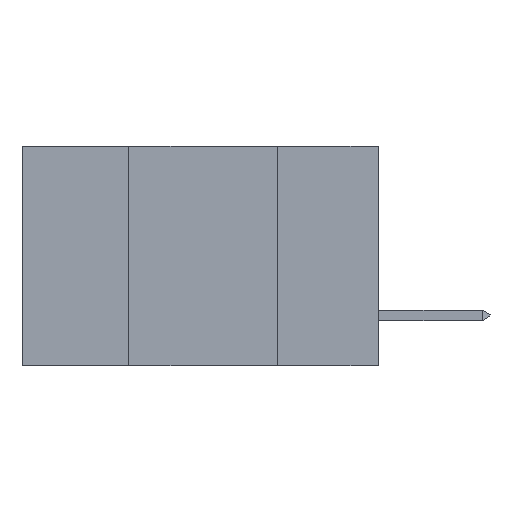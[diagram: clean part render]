
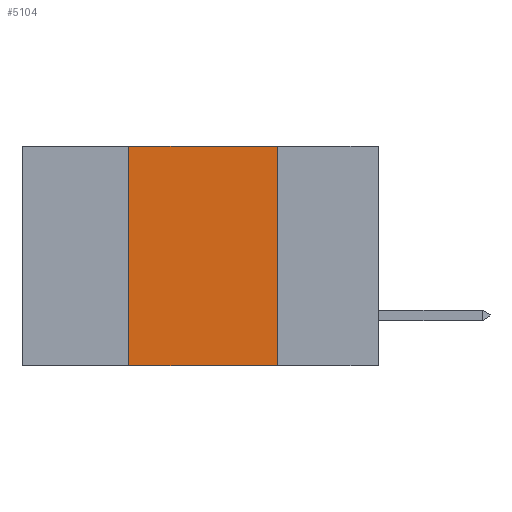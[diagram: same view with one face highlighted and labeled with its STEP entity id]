
A CAD part, left-side view. The second image highlights one B-rep face of the part: STEP entity #5104.
In plain terms, the highlighted planar face has unit normal (-1, 0, 0).
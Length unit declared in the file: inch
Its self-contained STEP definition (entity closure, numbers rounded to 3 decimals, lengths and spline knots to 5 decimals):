
#540 = EDGE_CURVE ( 'NONE', #7114, #6275, #2374, .T. ) ;
#1129 = AXIS2_PLACEMENT_3D ( 'NONE', #11163, #4843, #6060 ) ;
#2374 = LINE ( 'NONE', #8727, #5326 ) ;
#2601 = CARTESIAN_POINT ( 'NONE',  ( 0., 0.42, -0.37 ) ) ;
#2803 = CARTESIAN_POINT ( 'NONE',  ( 0., 0.17, -0.37 ) ) ;
#3100 = CARTESIAN_POINT ( 'NONE',  ( 0., 0.17, 0. ) ) ;
#3143 = DIRECTION ( 'NONE',  ( 0., -1., 0. ) ) ;
#3910 = DIRECTION ( 'NONE',  ( 0., 0., -1. ) ) ;
#4780 = VERTEX_POINT ( 'NONE', #3100 ) ;
#4843 = DIRECTION ( 'NONE',  ( 1., 0., 0. ) ) ;
#5104 = ADVANCED_FACE ( 'NONE', ( #5792 ), #13165, .F. ) ;
#5326 = VECTOR ( 'NONE', #11069, 39.37008 ) ;
#5466 = EDGE_CURVE ( 'NONE', #4780, #6275, #13154, .T. ) ;
#5792 = FACE_OUTER_BOUND ( 'NONE', #6506, .T. ) ;
#5858 = ORIENTED_EDGE ( 'NONE', *, *, #540, .T. ) ;
#6060 = DIRECTION ( 'NONE',  ( 0., 0., -1. ) ) ;
#6275 = VERTEX_POINT ( 'NONE', #13023 ) ;
#6387 = CARTESIAN_POINT ( 'NONE',  ( 0., 0.6, 0. ) ) ;
#6506 = EDGE_LOOP ( 'NONE', ( #10018, #6529, #9002, #5858 ) ) ;
#6529 = ORIENTED_EDGE ( 'NONE', *, *, #8451, .F. ) ;
#7114 = VERTEX_POINT ( 'NONE', #2601 ) ;
#7249 = CARTESIAN_POINT ( 'NONE',  ( 0., 0.42, -0.37 ) ) ;
#7506 = VERTEX_POINT ( 'NONE', #13211 ) ;
#8204 = LINE ( 'NONE', #6387, #9589 ) ;
#8451 = EDGE_CURVE ( 'NONE', #7506, #4780, #8204, .T. ) ;
#8727 = CARTESIAN_POINT ( 'NONE',  ( 0., 0.6, -0.37 ) ) ;
#9002 = ORIENTED_EDGE ( 'NONE', *, *, #12013, .F. ) ;
#9589 = VECTOR ( 'NONE', #3143, 39.37008 ) ;
#10018 = ORIENTED_EDGE ( 'NONE', *, *, #5466, .F. ) ;
#10231 = LINE ( 'NONE', #7249, #10305 ) ;
#10305 = VECTOR ( 'NONE', #12350, 39.37008 ) ;
#10861 = VECTOR ( 'NONE', #3910, 39.37008 ) ;
#11069 = DIRECTION ( 'NONE',  ( 0., -1., 0. ) ) ;
#11163 = CARTESIAN_POINT ( 'NONE',  ( 0., 0.6, 0. ) ) ;
#12013 = EDGE_CURVE ( 'NONE', #7114, #7506, #10231, .T. ) ;
#12350 = DIRECTION ( 'NONE',  ( 0., 0., 1. ) ) ;
#13023 = CARTESIAN_POINT ( 'NONE',  ( 0., 0.17, -0.37 ) ) ;
#13154 = LINE ( 'NONE', #2803, #10861 ) ;
#13165 = PLANE ( 'NONE',  #1129 ) ;
#13211 = CARTESIAN_POINT ( 'NONE',  ( 0., 0.42, 0. ) ) ;
